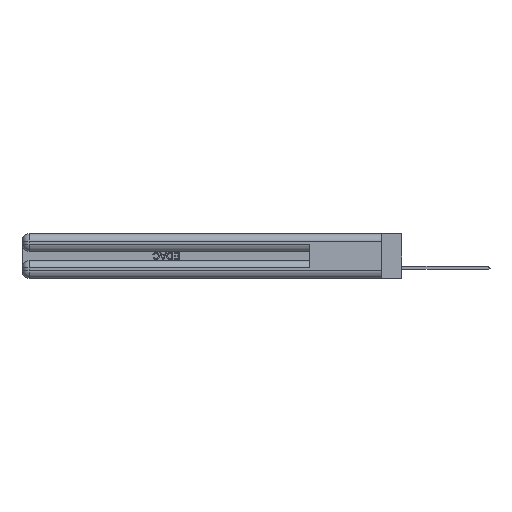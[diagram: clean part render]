
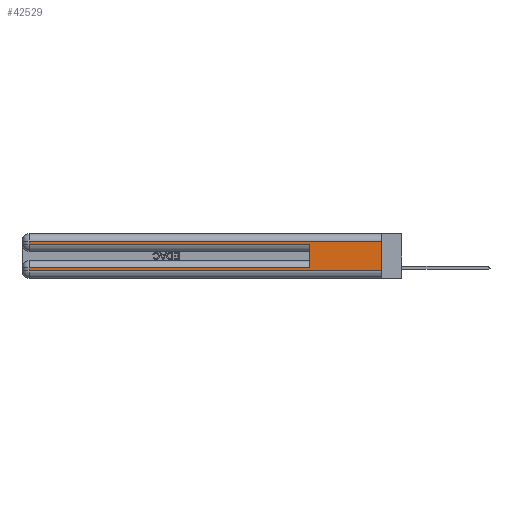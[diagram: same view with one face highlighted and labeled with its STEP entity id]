
A CAD part, left-side view. The second image highlights one B-rep face of the part: STEP entity #42529.
In plain terms, the highlighted planar face has unit normal (-1, 0, 0).
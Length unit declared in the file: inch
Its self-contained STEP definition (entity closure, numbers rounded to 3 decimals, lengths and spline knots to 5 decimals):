
#1740 = PLANE ( 'NONE',  #25962 ) ;
#1840 = CARTESIAN_POINT ( 'NONE',  ( 0., 0., 0.06 ) ) ;
#2384 = VECTOR ( 'NONE', #11637, 39.37008 ) ;
#2487 = LINE ( 'NONE', #51494, #27914 ) ;
#2498 = VECTOR ( 'NONE', #39445, 39.37008 ) ;
#5293 = DIRECTION ( 'NONE',  ( 1., 0., 0. ) ) ;
#5785 = EDGE_CURVE ( 'NONE', #21147, #11122, #8312, .T. ) ;
#6024 = CARTESIAN_POINT ( 'NONE',  ( 0., 0., 0.06 ) ) ;
#6467 = VECTOR ( 'NONE', #12841, 39.37008 ) ;
#7246 = CARTESIAN_POINT ( 'NONE',  ( 0., 0.6, 0.085 ) ) ;
#7297 = VERTEX_POINT ( 'NONE', #38128 ) ;
#7745 = CARTESIAN_POINT ( 'NONE',  ( 0., 0., 0.085 ) ) ;
#7948 = EDGE_CURVE ( 'NONE', #21147, #25492, #11342, .T. ) ;
#8312 = LINE ( 'NONE', #53862, #10347 ) ;
#9964 = CARTESIAN_POINT ( 'NONE',  ( 0., 2.94, 0.06 ) ) ;
#10347 = VECTOR ( 'NONE', #23533, 39.37008 ) ;
#10501 = EDGE_CURVE ( 'NONE', #28431, #11122, #25249, .T. ) ;
#10945 = EDGE_CURVE ( 'NONE', #7297, #28431, #17776, .T. ) ;
#11122 = VERTEX_POINT ( 'NONE', #1840 ) ;
#11342 = LINE ( 'NONE', #32076, #18695 ) ;
#11637 = DIRECTION ( 'NONE',  ( 0., 1., 0. ) ) ;
#12035 = VERTEX_POINT ( 'NONE', #36932 ) ;
#12841 = DIRECTION ( 'NONE',  ( 0., 0., -1. ) ) ;
#13442 = ORIENTED_EDGE ( 'NONE', *, *, #7948, .T. ) ;
#14632 = FACE_OUTER_BOUND ( 'NONE', #29829, .T. ) ;
#17776 = LINE ( 'NONE', #46556, #6467 ) ;
#18424 = VERTEX_POINT ( 'NONE', #7246 ) ;
#18695 = VECTOR ( 'NONE', #45142, 39.37008 ) ;
#21147 = VERTEX_POINT ( 'NONE', #36187 ) ;
#21858 = ORIENTED_EDGE ( 'NONE', *, *, #23217, .T. ) ;
#22546 = ORIENTED_EDGE ( 'NONE', *, *, #10945, .T. ) ;
#23067 = DIRECTION ( 'NONE',  ( 0., 0., -1. ) ) ;
#23217 = EDGE_CURVE ( 'NONE', #25492, #12035, #35102, .T. ) ;
#23533 = DIRECTION ( 'NONE',  ( 0., 0., -1. ) ) ;
#23551 = EDGE_CURVE ( 'NONE', #18424, #53382, #2487, .T. ) ;
#25118 = CARTESIAN_POINT ( 'NONE',  ( 0., 0., 0.285 ) ) ;
#25249 = LINE ( 'NONE', #6024, #2498 ) ;
#25492 = VERTEX_POINT ( 'NONE', #29746 ) ;
#25674 = DIRECTION ( 'NONE',  ( 0., 0., 1. ) ) ;
#25962 = AXIS2_PLACEMENT_3D ( 'NONE', #31654, #5293, #35936 ) ;
#27914 = VECTOR ( 'NONE', #25674, 39.37008 ) ;
#28431 = VERTEX_POINT ( 'NONE', #9964 ) ;
#29209 = DIRECTION ( 'NONE',  ( 0., -1., 0. ) ) ;
#29746 = CARTESIAN_POINT ( 'NONE',  ( 0., 2.94, 0.31 ) ) ;
#29829 = EDGE_LOOP ( 'NONE', ( #49029, #13442, #21858, #42427, #42623, #32941, #22546, #53548 ) ) ;
#31654 = CARTESIAN_POINT ( 'NONE',  ( 0., 0., 0.37 ) ) ;
#32076 = CARTESIAN_POINT ( 'NONE',  ( 0., 0., 0.31 ) ) ;
#32941 = ORIENTED_EDGE ( 'NONE', *, *, #35967, .T. ) ;
#35102 = LINE ( 'NONE', #44001, #46507 ) ;
#35936 = DIRECTION ( 'NONE',  ( 0., 0., -1. ) ) ;
#35967 = EDGE_CURVE ( 'NONE', #18424, #7297, #41140, .T. ) ;
#36187 = CARTESIAN_POINT ( 'NONE',  ( 0., 0., 0.31 ) ) ;
#36706 = VECTOR ( 'NONE', #29209, 39.37008 ) ;
#36932 = CARTESIAN_POINT ( 'NONE',  ( 0., 2.94, 0.285 ) ) ;
#38128 = CARTESIAN_POINT ( 'NONE',  ( 0., 2.94, 0.085 ) ) ;
#39445 = DIRECTION ( 'NONE',  ( 0., -1., 0. ) ) ;
#41140 = LINE ( 'NONE', #7745, #2384 ) ;
#42427 = ORIENTED_EDGE ( 'NONE', *, *, #47690, .T. ) ;
#42529 = ADVANCED_FACE ( 'NONE', ( #14632 ), #1740, .F. ) ;
#42623 = ORIENTED_EDGE ( 'NONE', *, *, #23551, .F. ) ;
#44001 = CARTESIAN_POINT ( 'NONE',  ( 0., 2.94, 0.37 ) ) ;
#45142 = DIRECTION ( 'NONE',  ( 0., 1., 0. ) ) ;
#46507 = VECTOR ( 'NONE', #23067, 39.37008 ) ;
#46556 = CARTESIAN_POINT ( 'NONE',  ( 0., 2.94, 0.37 ) ) ;
#47690 = EDGE_CURVE ( 'NONE', #12035, #53382, #54146, .T. ) ;
#49029 = ORIENTED_EDGE ( 'NONE', *, *, #5785, .F. ) ;
#51494 = CARTESIAN_POINT ( 'NONE',  ( 0., 0.6, 0.145 ) ) ;
#53382 = VERTEX_POINT ( 'NONE', #54149 ) ;
#53548 = ORIENTED_EDGE ( 'NONE', *, *, #10501, .T. ) ;
#53862 = CARTESIAN_POINT ( 'NONE',  ( 0., 0., 0.37 ) ) ;
#54146 = LINE ( 'NONE', #25118, #36706 ) ;
#54149 = CARTESIAN_POINT ( 'NONE',  ( 0., 0.6, 0.285 ) ) ;
